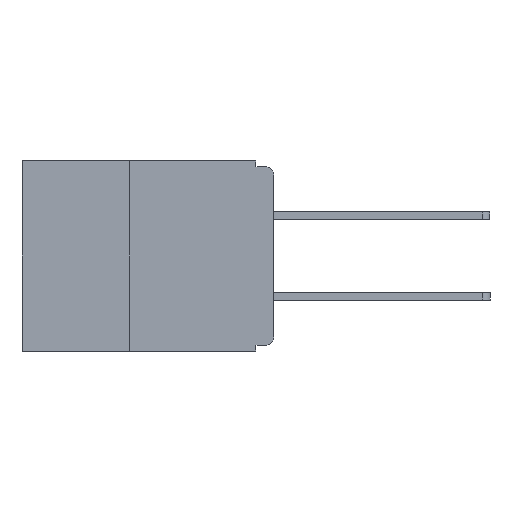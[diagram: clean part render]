
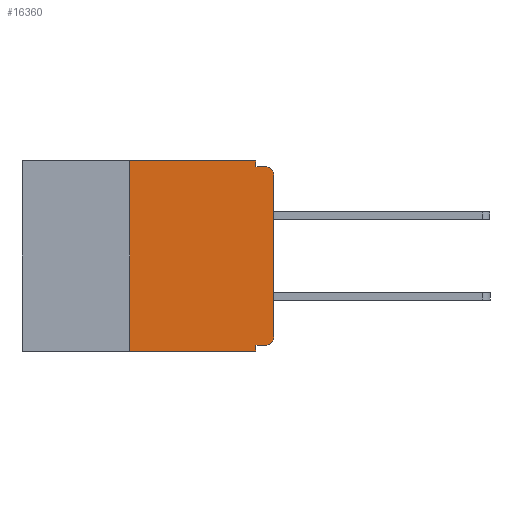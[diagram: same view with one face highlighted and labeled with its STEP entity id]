
A CAD part, left-side view. The second image highlights one B-rep face of the part: STEP entity #16360.
In plain terms, the highlighted planar face has unit normal (-1, 0, 0).
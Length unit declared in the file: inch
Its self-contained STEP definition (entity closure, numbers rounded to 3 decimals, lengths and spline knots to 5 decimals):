
#134 = DIRECTION ( 'NONE',  ( 0., -1., 0. ) ) ;
#413 = VERTEX_POINT ( 'NONE', #10059 ) ;
#480 = CARTESIAN_POINT ( 'NONE',  ( 0., 0., 0. ) ) ;
#514 = LINE ( 'NONE', #20357, #22252 ) ;
#623 = DIRECTION ( 'NONE',  ( 0., 0., 1. ) ) ;
#747 = VECTOR ( 'NONE', #23414, 39.37008 ) ;
#789 = VERTEX_POINT ( 'NONE', #23818 ) ;
#1227 = DIRECTION ( 'NONE',  ( 0., -1., 0. ) ) ;
#1233 = EDGE_CURVE ( 'NONE', #17328, #20883, #3919, .T. ) ;
#1293 = CARTESIAN_POINT ( 'NONE',  ( 0., 0.031, -0.01 ) ) ;
#1784 = VECTOR ( 'NONE', #15725, 39.37008 ) ;
#1816 = ORIENTED_EDGE ( 'NONE', *, *, #6382, .T. ) ;
#1918 = DIRECTION ( 'NONE',  ( 0., 0., -1. ) ) ;
#2508 = CIRCLE ( 'NONE', #23878, 0.015 ) ;
#2812 = CARTESIAN_POINT ( 'NONE',  ( 0., 0., -0.305 ) ) ;
#3406 = ORIENTED_EDGE ( 'NONE', *, *, #20821, .F. ) ;
#3557 = VECTOR ( 'NONE', #1227, 39.37008 ) ;
#3906 = LINE ( 'NONE', #23608, #15196 ) ;
#3919 = CIRCLE ( 'NONE', #15607, 0.015 ) ;
#4039 = ORIENTED_EDGE ( 'NONE', *, *, #21034, .F. ) ;
#4389 = CARTESIAN_POINT ( 'NONE',  ( 0., 0.015, -0.01 ) ) ;
#6187 = CARTESIAN_POINT ( 'NONE',  ( 0., 0.031, 0. ) ) ;
#6382 = EDGE_CURVE ( 'NONE', #20883, #10029, #26875, .T. ) ;
#6796 = ORIENTED_EDGE ( 'NONE', *, *, #15635, .F. ) ;
#6933 = EDGE_CURVE ( 'NONE', #10029, #18906, #2508, .T. ) ;
#7445 = LINE ( 'NONE', #15647, #1784 ) ;
#7853 = DIRECTION ( 'NONE',  ( 0., 0., -1. ) ) ;
#8274 = DIRECTION ( 'NONE',  ( 0., 0., -1. ) ) ;
#8333 = DIRECTION ( 'NONE',  ( -1., 0., 0. ) ) ;
#8394 = CARTESIAN_POINT ( 'NONE',  ( 0., 0.015, -0.305 ) ) ;
#8554 = CARTESIAN_POINT ( 'NONE',  ( 0., 0.031, 0. ) ) ;
#9483 = VECTOR ( 'NONE', #623, 39.37008 ) ;
#9603 = ORIENTED_EDGE ( 'NONE', *, *, #1233, .T. ) ;
#9818 = AXIS2_PLACEMENT_3D ( 'NONE', #11869, #26522, #13998 ) ;
#9845 = LINE ( 'NONE', #22224, #3557 ) ;
#10029 = VERTEX_POINT ( 'NONE', #17736 ) ;
#10059 = CARTESIAN_POINT ( 'NONE',  ( 0., 0.25, 0. ) ) ;
#10348 = LINE ( 'NONE', #14944, #20875 ) ;
#11110 = VERTEX_POINT ( 'NONE', #8554 ) ;
#11160 = EDGE_CURVE ( 'NONE', #17328, #789, #17610, .T. ) ;
#11869 = CARTESIAN_POINT ( 'NONE',  ( 0., 0.437, 0. ) ) ;
#11900 = ORIENTED_EDGE ( 'NONE', *, *, #22206, .F. ) ;
#12700 = EDGE_LOOP ( 'NONE', ( #1816, #18209, #4039, #11900, #6796, #3406, #18034, #22392, #17461, #9603 ) ) ;
#13092 = VECTOR ( 'NONE', #1918, 39.37008 ) ;
#13684 = CARTESIAN_POINT ( 'NONE',  ( 0., 0.031, -0.33 ) ) ;
#13936 = CARTESIAN_POINT ( 'NONE',  ( 0., 0.25, -0.33 ) ) ;
#13998 = DIRECTION ( 'NONE',  ( 0., 0., -1. ) ) ;
#14944 = CARTESIAN_POINT ( 'NONE',  ( 0., 0.437, -0.33 ) ) ;
#15002 = CARTESIAN_POINT ( 'NONE',  ( 0., 0.015, -0.32 ) ) ;
#15196 = VECTOR ( 'NONE', #25725, 39.37008 ) ;
#15241 = EDGE_CURVE ( 'NONE', #789, #21912, #514, .T. ) ;
#15607 = AXIS2_PLACEMENT_3D ( 'NONE', #8394, #8333, #8274 ) ;
#15635 = EDGE_CURVE ( 'NONE', #413, #11110, #7445, .T. ) ;
#15647 = CARTESIAN_POINT ( 'NONE',  ( 0., 0.437, 0. ) ) ;
#15725 = DIRECTION ( 'NONE',  ( 0., -1., 0. ) ) ;
#15727 = VERTEX_POINT ( 'NONE', #13936 ) ;
#16360 = ADVANCED_FACE ( 'NONE', ( #21232 ), #24413, .F. ) ;
#16614 = EDGE_CURVE ( 'NONE', #15727, #21912, #10348, .T. ) ;
#17123 = CARTESIAN_POINT ( 'NONE',  ( 0., 0., -0.32 ) ) ;
#17328 = VERTEX_POINT ( 'NONE', #15002 ) ;
#17461 = ORIENTED_EDGE ( 'NONE', *, *, #11160, .F. ) ;
#17610 = LINE ( 'NONE', #17123, #747 ) ;
#17736 = CARTESIAN_POINT ( 'NONE',  ( 0., 0., -0.025 ) ) ;
#18034 = ORIENTED_EDGE ( 'NONE', *, *, #16614, .T. ) ;
#18209 = ORIENTED_EDGE ( 'NONE', *, *, #6933, .T. ) ;
#18890 = DIRECTION ( 'NONE',  ( 0., 0., -1. ) ) ;
#18906 = VERTEX_POINT ( 'NONE', #4389 ) ;
#18945 = DIRECTION ( 'NONE',  ( -1., 0., 0. ) ) ;
#18971 = CARTESIAN_POINT ( 'NONE',  ( 0., 0.015, -0.025 ) ) ;
#19324 = LINE ( 'NONE', #6187, #13092 ) ;
#20357 = CARTESIAN_POINT ( 'NONE',  ( 0., 0.031, -0.33 ) ) ;
#20821 = EDGE_CURVE ( 'NONE', #15727, #413, #3906, .T. ) ;
#20875 = VECTOR ( 'NONE', #134, 39.37008 ) ;
#20883 = VERTEX_POINT ( 'NONE', #2812 ) ;
#21034 = EDGE_CURVE ( 'NONE', #23828, #18906, #9845, .T. ) ;
#21232 = FACE_OUTER_BOUND ( 'NONE', #12700, .T. ) ;
#21912 = VERTEX_POINT ( 'NONE', #13684 ) ;
#22206 = EDGE_CURVE ( 'NONE', #11110, #23828, #19324, .T. ) ;
#22224 = CARTESIAN_POINT ( 'NONE',  ( 0., 0., -0.01 ) ) ;
#22252 = VECTOR ( 'NONE', #7853, 39.37008 ) ;
#22392 = ORIENTED_EDGE ( 'NONE', *, *, #15241, .F. ) ;
#23414 = DIRECTION ( 'NONE',  ( 0., 1., 0. ) ) ;
#23608 = CARTESIAN_POINT ( 'NONE',  ( 0., 0.25, -0.33 ) ) ;
#23818 = CARTESIAN_POINT ( 'NONE',  ( 0., 0.031, -0.32 ) ) ;
#23828 = VERTEX_POINT ( 'NONE', #1293 ) ;
#23878 = AXIS2_PLACEMENT_3D ( 'NONE', #18971, #18945, #18890 ) ;
#24413 = PLANE ( 'NONE',  #9818 ) ;
#25725 = DIRECTION ( 'NONE',  ( 0., 0., 1. ) ) ;
#26522 = DIRECTION ( 'NONE',  ( 1., 0., 0. ) ) ;
#26875 = LINE ( 'NONE', #480, #9483 ) ;
